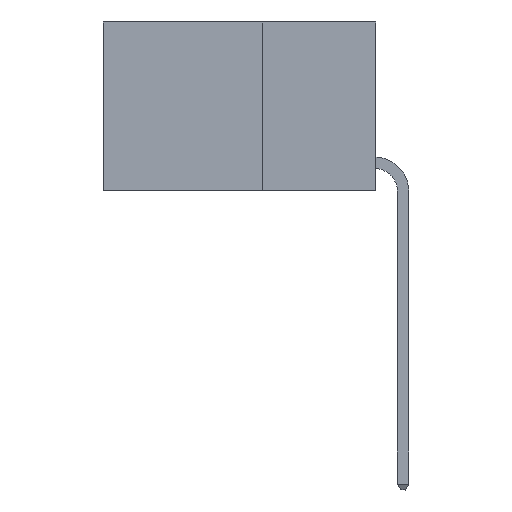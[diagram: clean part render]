
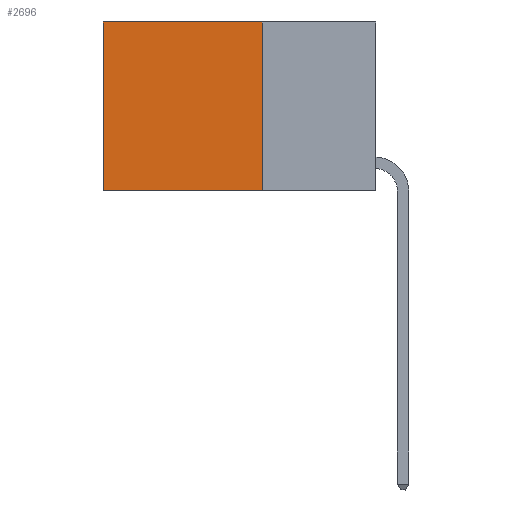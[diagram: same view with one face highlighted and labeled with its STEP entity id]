
A CAD part, left-side view. The second image highlights one B-rep face of the part: STEP entity #2696.
In plain terms, the highlighted planar face has unit normal (-1, 0, 0).
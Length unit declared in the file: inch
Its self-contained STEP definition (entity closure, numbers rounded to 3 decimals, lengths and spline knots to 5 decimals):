
#2696 = ADVANCED_FACE ( 'NONE', ( #24039 ), #11758, .F. ) ;
#2772 = DIRECTION ( 'NONE',  ( 0., 0., -1. ) ) ;
#2971 = LINE ( 'NONE', #4941, #17463 ) ;
#3445 = EDGE_CURVE ( 'NONE', #21873, #24054, #11148, .T. ) ;
#3683 = DIRECTION ( 'NONE',  ( 0., 1., 0. ) ) ;
#4219 = DIRECTION ( 'NONE',  ( 1., 0., 0. ) ) ;
#4306 = EDGE_CURVE ( 'NONE', #24054, #22892, #16984, .T. ) ;
#4824 = EDGE_LOOP ( 'NONE', ( #19417, #11318, #17253, #6031 ) ) ;
#4941 = CARTESIAN_POINT ( 'NONE',  ( 0.2625, 0.6, 0. ) ) ;
#5896 = DIRECTION ( 'NONE',  ( 0., 1., 0. ) ) ;
#6031 = ORIENTED_EDGE ( 'NONE', *, *, #15368, .T. ) ;
#6930 = VECTOR ( 'NONE', #5896, 39.37008 ) ;
#7562 = CARTESIAN_POINT ( 'NONE',  ( 0.2625, 0.25, 0. ) ) ;
#8032 = LINE ( 'NONE', #13087, #12464 ) ;
#10470 = CARTESIAN_POINT ( 'NONE',  ( 0.2625, 0.6, -0.37 ) ) ;
#10734 = CARTESIAN_POINT ( 'NONE',  ( 0.2625, 0.25, -0.37 ) ) ;
#11148 = LINE ( 'NONE', #23421, #20552 ) ;
#11318 = ORIENTED_EDGE ( 'NONE', *, *, #4306, .F. ) ;
#11758 = PLANE ( 'NONE',  #15469 ) ;
#12464 = VECTOR ( 'NONE', #3683, 39.37008 ) ;
#13087 = CARTESIAN_POINT ( 'NONE',  ( 0.2625, 0.25, 0. ) ) ;
#15368 = EDGE_CURVE ( 'NONE', #21873, #16070, #8032, .T. ) ;
#15469 = AXIS2_PLACEMENT_3D ( 'NONE', #22963, #4219, #17441 ) ;
#16070 = VERTEX_POINT ( 'NONE', #16859 ) ;
#16339 = DIRECTION ( 'NONE',  ( 0., 0., -1. ) ) ;
#16566 = EDGE_CURVE ( 'NONE', #16070, #22892, #2971, .T. ) ;
#16859 = CARTESIAN_POINT ( 'NONE',  ( 0.2625, 0.6, 0. ) ) ;
#16984 = LINE ( 'NONE', #19002, #6930 ) ;
#17253 = ORIENTED_EDGE ( 'NONE', *, *, #3445, .F. ) ;
#17441 = DIRECTION ( 'NONE',  ( 0., 0., -1. ) ) ;
#17463 = VECTOR ( 'NONE', #16339, 39.37008 ) ;
#19002 = CARTESIAN_POINT ( 'NONE',  ( 0.2625, 0.25, -0.37 ) ) ;
#19417 = ORIENTED_EDGE ( 'NONE', *, *, #16566, .T. ) ;
#20552 = VECTOR ( 'NONE', #2772, 39.37008 ) ;
#21873 = VERTEX_POINT ( 'NONE', #7562 ) ;
#22892 = VERTEX_POINT ( 'NONE', #10470 ) ;
#22963 = CARTESIAN_POINT ( 'NONE',  ( 0.2625, 0.25, 0. ) ) ;
#23421 = CARTESIAN_POINT ( 'NONE',  ( 0.2625, 0.25, 0. ) ) ;
#24039 = FACE_OUTER_BOUND ( 'NONE', #4824, .T. ) ;
#24054 = VERTEX_POINT ( 'NONE', #10734 ) ;
